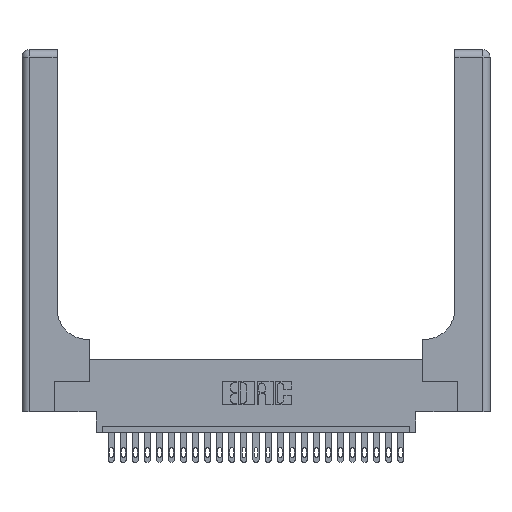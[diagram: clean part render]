
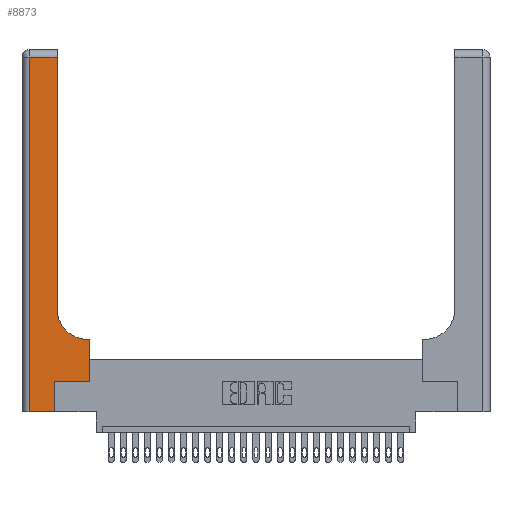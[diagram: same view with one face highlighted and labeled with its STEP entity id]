
A CAD part, top view. The second image highlights one B-rep face of the part: STEP entity #8873.
In plain terms, the highlighted planar face has unit normal (0, 0, 1).
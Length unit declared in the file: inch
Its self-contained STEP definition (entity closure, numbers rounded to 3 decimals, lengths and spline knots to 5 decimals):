
#290 = VECTOR ( 'NONE', #15218, 39.37008 ) ;
#1002 = VERTEX_POINT ( 'NONE', #15453 ) ;
#1031 = PLANE ( 'NONE',  #11717 ) ;
#1241 = EDGE_CURVE ( 'NONE', #13951, #14684, #21697, .T. ) ;
#1361 = CARTESIAN_POINT ( 'NONE',  ( 0.2915, 0.6, 0.37 ) ) ;
#1682 = CARTESIAN_POINT ( 'NONE',  ( 0.06, 3., 0.37 ) ) ;
#2279 = CARTESIAN_POINT ( 'NONE',  ( 0.5415, 0.85, 0.37 ) ) ;
#2777 = CIRCLE ( 'NONE', #3202, 0.25 ) ;
#3090 = CARTESIAN_POINT ( 'NONE',  ( 0., 3., 0.37 ) ) ;
#3202 = AXIS2_PLACEMENT_3D ( 'NONE', #2279, #18728, #6575 ) ;
#3427 = CARTESIAN_POINT ( 'NONE',  ( 0.269, 0.25, 0.37 ) ) ;
#5574 = LINE ( 'NONE', #18667, #7853 ) ;
#5845 = ORIENTED_EDGE ( 'NONE', *, *, #18439, .T. ) ;
#5937 = VERTEX_POINT ( 'NONE', #9840 ) ;
#6082 = EDGE_CURVE ( 'NONE', #14680, #5937, #8975, .T. ) ;
#6532 = VERTEX_POINT ( 'NONE', #3427 ) ;
#6575 = DIRECTION ( 'NONE',  ( 1., 0., 0. ) ) ;
#6607 = LINE ( 'NONE', #16383, #9834 ) ;
#6635 = CARTESIAN_POINT ( 'NONE',  ( 0.5585, 0.6, 0.37 ) ) ;
#6759 = LINE ( 'NONE', #8967, #20395 ) ;
#7202 = DIRECTION ( 'NONE',  ( -1., 0., 0. ) ) ;
#7248 = ORIENTED_EDGE ( 'NONE', *, *, #10945, .T. ) ;
#7853 = VECTOR ( 'NONE', #25901, 39.37008 ) ;
#8429 = VERTEX_POINT ( 'NONE', #17021 ) ;
#8873 = ADVANCED_FACE ( 'NONE', ( #10197 ), #1031, .F. ) ;
#8967 = CARTESIAN_POINT ( 'NONE',  ( 0.2915, 3., 0.37 ) ) ;
#8975 = LINE ( 'NONE', #1682, #15298 ) ;
#9797 = EDGE_CURVE ( 'NONE', #1002, #14563, #2777, .T. ) ;
#9834 = VECTOR ( 'NONE', #18264, 39.37008 ) ;
#9840 = CARTESIAN_POINT ( 'NONE',  ( 0.06, 0., 0.37 ) ) ;
#10043 = CARTESIAN_POINT ( 'NONE',  ( 0., 0., 0.37 ) ) ;
#10197 = FACE_OUTER_BOUND ( 'NONE', #19608, .T. ) ;
#10242 = ORIENTED_EDGE ( 'NONE', *, *, #24643, .T. ) ;
#10866 = LINE ( 'NONE', #1361, #290 ) ;
#10945 = EDGE_CURVE ( 'NONE', #6532, #13951, #5574, .T. ) ;
#11177 = DIRECTION ( 'NONE',  ( 0., 1., 0. ) ) ;
#11220 = CARTESIAN_POINT ( 'NONE',  ( 0.5585, 0.25, 0.37 ) ) ;
#11717 = AXIS2_PLACEMENT_3D ( 'NONE', #3090, #17297, #15887 ) ;
#12688 = ORIENTED_EDGE ( 'NONE', *, *, #1241, .T. ) ;
#13145 = VECTOR ( 'NONE', #19294, 39.37008 ) ;
#13413 = CARTESIAN_POINT ( 'NONE',  ( 0.2915, 0.85, 0.37 ) ) ;
#13951 = VERTEX_POINT ( 'NONE', #24193 ) ;
#14255 = EDGE_CURVE ( 'NONE', #5937, #20356, #22176, .T. ) ;
#14563 = VERTEX_POINT ( 'NONE', #13413 ) ;
#14680 = VERTEX_POINT ( 'NONE', #14798 ) ;
#14684 = VERTEX_POINT ( 'NONE', #6635 ) ;
#14691 = LINE ( 'NONE', #17100, #18468 ) ;
#14798 = CARTESIAN_POINT ( 'NONE',  ( 0.06, 2.94, 0.37 ) ) ;
#15218 = DIRECTION ( 'NONE',  ( -1., 0., 0. ) ) ;
#15298 = VECTOR ( 'NONE', #25828, 39.37008 ) ;
#15453 = CARTESIAN_POINT ( 'NONE',  ( 0.5415, 0.6, 0.37 ) ) ;
#15887 = DIRECTION ( 'NONE',  ( -1., 0., 0. ) ) ;
#16126 = DIRECTION ( 'NONE',  ( 1., 0., 0. ) ) ;
#16383 = CARTESIAN_POINT ( 'NONE',  ( 0.269, 0., 0.37 ) ) ;
#16869 = CARTESIAN_POINT ( 'NONE',  ( 0.269, 0., 0.37 ) ) ;
#17021 = CARTESIAN_POINT ( 'NONE',  ( 0.2915, 2.94, 0.37 ) ) ;
#17100 = CARTESIAN_POINT ( 'NONE',  ( 0., 2.94, 0.37 ) ) ;
#17297 = DIRECTION ( 'NONE',  ( 0., 0., -1. ) ) ;
#17386 = ORIENTED_EDGE ( 'NONE', *, *, #9797, .T. ) ;
#18264 = DIRECTION ( 'NONE',  ( 0., 1., 0. ) ) ;
#18417 = EDGE_CURVE ( 'NONE', #14563, #8429, #6759, .T. ) ;
#18439 = EDGE_CURVE ( 'NONE', #8429, #14680, #14691, .T. ) ;
#18468 = VECTOR ( 'NONE', #7202, 39.37008 ) ;
#18667 = CARTESIAN_POINT ( 'NONE',  ( 0.269, 0.25, 0.37 ) ) ;
#18728 = DIRECTION ( 'NONE',  ( 0., 0., -1. ) ) ;
#19294 = DIRECTION ( 'NONE',  ( 0., 1., 0. ) ) ;
#19608 = EDGE_LOOP ( 'NONE', ( #19627, #5845, #25149, #25542, #10242, #7248, #12688, #21549, #17386 ) ) ;
#19627 = ORIENTED_EDGE ( 'NONE', *, *, #18417, .T. ) ;
#20356 = VERTEX_POINT ( 'NONE', #16869 ) ;
#20395 = VECTOR ( 'NONE', #11177, 39.37008 ) ;
#21549 = ORIENTED_EDGE ( 'NONE', *, *, #21735, .T. ) ;
#21697 = LINE ( 'NONE', #11220, #13145 ) ;
#21735 = EDGE_CURVE ( 'NONE', #14684, #1002, #10866, .T. ) ;
#22176 = LINE ( 'NONE', #10043, #22809 ) ;
#22809 = VECTOR ( 'NONE', #16126, 39.37008 ) ;
#24193 = CARTESIAN_POINT ( 'NONE',  ( 0.5585, 0.25, 0.37 ) ) ;
#24643 = EDGE_CURVE ( 'NONE', #20356, #6532, #6607, .T. ) ;
#25149 = ORIENTED_EDGE ( 'NONE', *, *, #6082, .T. ) ;
#25542 = ORIENTED_EDGE ( 'NONE', *, *, #14255, .T. ) ;
#25828 = DIRECTION ( 'NONE',  ( 0., -1., 0. ) ) ;
#25901 = DIRECTION ( 'NONE',  ( 1., 0., 0. ) ) ;
